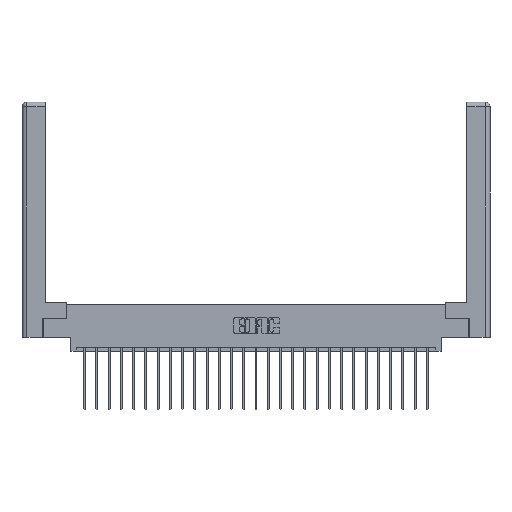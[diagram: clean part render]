
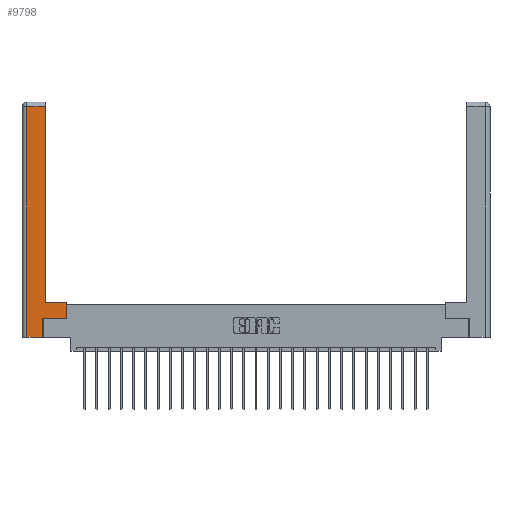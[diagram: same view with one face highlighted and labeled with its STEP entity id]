
A CAD part, top view. The second image highlights one B-rep face of the part: STEP entity #9798.
In plain terms, the highlighted planar face has unit normal (0, 0, 1).
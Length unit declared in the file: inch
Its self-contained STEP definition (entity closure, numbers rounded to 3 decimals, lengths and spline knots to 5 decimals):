
#91 = CARTESIAN_POINT ( 'NONE',  ( 0., 0., 0. ) ) ;
#743 = DIRECTION ( 'NONE',  ( 0., 0., -1. ) ) ;
#965 = ORIENTED_EDGE ( 'NONE', *, *, #21937, .T. ) ;
#1460 = LINE ( 'NONE', #15716, #26235 ) ;
#1691 = DIRECTION ( 'NONE',  ( 0., 1., 0. ) ) ;
#2757 = LINE ( 'NONE', #3236, #9259 ) ;
#3043 = EDGE_LOOP ( 'NONE', ( #965, #6836, #21656, #7820, #9570, #3438, #24264, #17872 ) ) ;
#3236 = CARTESIAN_POINT ( 'NONE',  ( 0.0615, 0., 0. ) ) ;
#3438 = ORIENTED_EDGE ( 'NONE', *, *, #10353, .T. ) ;
#4096 = VERTEX_POINT ( 'NONE', #21733 ) ;
#4496 = VECTOR ( 'NONE', #19420, 39.37008 ) ;
#5765 = VERTEX_POINT ( 'NONE', #13412 ) ;
#5772 = DIRECTION ( 'NONE',  ( -1., 0., 0. ) ) ;
#6086 = LINE ( 'NONE', #8208, #9366 ) ;
#6336 = AXIS2_PLACEMENT_3D ( 'NONE', #91, #743, #14778 ) ;
#6836 = ORIENTED_EDGE ( 'NONE', *, *, #21393, .T. ) ;
#7820 = ORIENTED_EDGE ( 'NONE', *, *, #21096, .T. ) ;
#8208 = CARTESIAN_POINT ( 'NONE',  ( 0.295, 0.45, 0. ) ) ;
#8955 = CARTESIAN_POINT ( 'NONE',  ( 0.0615, 2.94, 0. ) ) ;
#9259 = VECTOR ( 'NONE', #26069, 39.37008 ) ;
#9366 = VECTOR ( 'NONE', #5772, 39.37008 ) ;
#9570 = ORIENTED_EDGE ( 'NONE', *, *, #25300, .T. ) ;
#9605 = DIRECTION ( 'NONE',  ( 0., 1., 0. ) ) ;
#9642 = VERTEX_POINT ( 'NONE', #14204 ) ;
#9798 = ADVANCED_FACE ( 'NONE', ( #25999 ), #12511, .F. ) ;
#10353 = EDGE_CURVE ( 'NONE', #4096, #22902, #25969, .T. ) ;
#10365 = VECTOR ( 'NONE', #22446, 39.37008 ) ;
#10891 = LINE ( 'NONE', #20714, #23241 ) ;
#12511 = PLANE ( 'NONE',  #6336 ) ;
#12529 = CARTESIAN_POINT ( 'NONE',  ( 0.0615, 0., 0. ) ) ;
#12697 = CARTESIAN_POINT ( 'NONE',  ( 0.295, 2.94, 0. ) ) ;
#13289 = CARTESIAN_POINT ( 'NONE',  ( 0.265, 0., 0. ) ) ;
#13412 = CARTESIAN_POINT ( 'NONE',  ( 0.295, 0.45, 0. ) ) ;
#13645 = VERTEX_POINT ( 'NONE', #13289 ) ;
#14204 = CARTESIAN_POINT ( 'NONE',  ( 0.565, 0.45, 0. ) ) ;
#14605 = LINE ( 'NONE', #8955, #4496 ) ;
#14778 = DIRECTION ( 'NONE',  ( -1., 0., 0. ) ) ;
#15716 = CARTESIAN_POINT ( 'NONE',  ( 0.265, 0.245, 0. ) ) ;
#16464 = CARTESIAN_POINT ( 'NONE',  ( 0.565, 0.245, 0. ) ) ;
#16752 = VERTEX_POINT ( 'NONE', #12529 ) ;
#17842 = CARTESIAN_POINT ( 'NONE',  ( 0.565, 0.245, 0. ) ) ;
#17872 = ORIENTED_EDGE ( 'NONE', *, *, #24280, .T. ) ;
#18724 = VERTEX_POINT ( 'NONE', #12697 ) ;
#18939 = VERTEX_POINT ( 'NONE', #23562 ) ;
#19420 = DIRECTION ( 'NONE',  ( -1., 0., 0. ) ) ;
#19422 = VECTOR ( 'NONE', #24478, 39.37008 ) ;
#20055 = CARTESIAN_POINT ( 'NONE',  ( 0.265, 0., 0. ) ) ;
#20714 = CARTESIAN_POINT ( 'NONE',  ( 0.565, 0.45, 0. ) ) ;
#21096 = EDGE_CURVE ( 'NONE', #16752, #13645, #25392, .T. ) ;
#21393 = EDGE_CURVE ( 'NONE', #18724, #18939, #14605, .T. ) ;
#21656 = ORIENTED_EDGE ( 'NONE', *, *, #26126, .T. ) ;
#21733 = CARTESIAN_POINT ( 'NONE',  ( 0.265, 0.245, 0. ) ) ;
#21937 = EDGE_CURVE ( 'NONE', #5765, #18724, #26001, .T. ) ;
#22446 = DIRECTION ( 'NONE',  ( 1., 0., 0. ) ) ;
#22902 = VERTEX_POINT ( 'NONE', #17842 ) ;
#23241 = VECTOR ( 'NONE', #1691, 39.37008 ) ;
#23562 = CARTESIAN_POINT ( 'NONE',  ( 0.0615, 2.94, 0. ) ) ;
#24264 = ORIENTED_EDGE ( 'NONE', *, *, #25904, .T. ) ;
#24280 = EDGE_CURVE ( 'NONE', #9642, #5765, #6086, .T. ) ;
#24478 = DIRECTION ( 'NONE',  ( 1., 0., 0. ) ) ;
#25011 = VECTOR ( 'NONE', #25437, 39.37008 ) ;
#25063 = CARTESIAN_POINT ( 'NONE',  ( 0.295, 3., 0. ) ) ;
#25300 = EDGE_CURVE ( 'NONE', #13645, #4096, #1460, .T. ) ;
#25392 = LINE ( 'NONE', #20055, #10365 ) ;
#25437 = DIRECTION ( 'NONE',  ( 0., 1., 0. ) ) ;
#25904 = EDGE_CURVE ( 'NONE', #22902, #9642, #10891, .T. ) ;
#25969 = LINE ( 'NONE', #16464, #19422 ) ;
#25999 = FACE_OUTER_BOUND ( 'NONE', #3043, .T. ) ;
#26001 = LINE ( 'NONE', #25063, #25011 ) ;
#26069 = DIRECTION ( 'NONE',  ( 0., -1., 0. ) ) ;
#26126 = EDGE_CURVE ( 'NONE', #18939, #16752, #2757, .T. ) ;
#26235 = VECTOR ( 'NONE', #9605, 39.37008 ) ;
